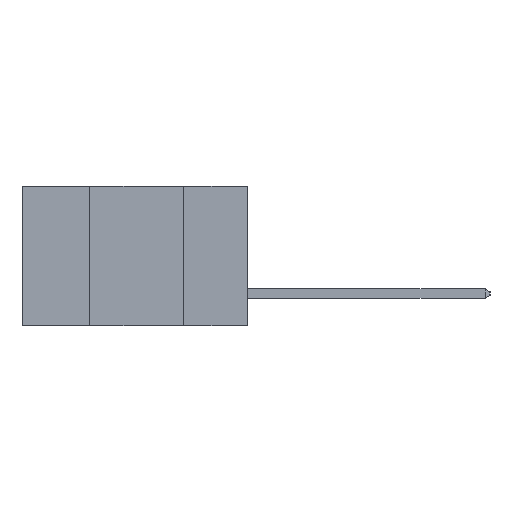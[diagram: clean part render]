
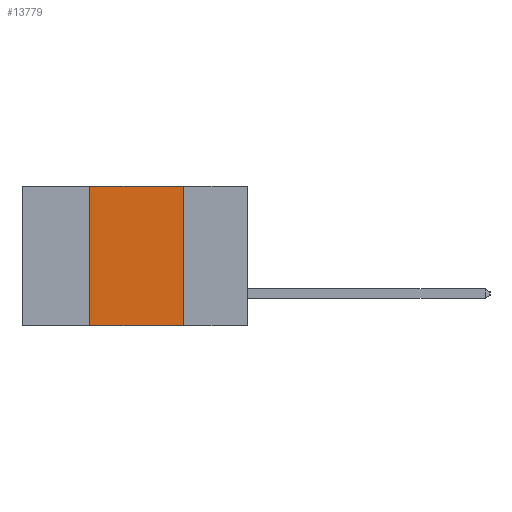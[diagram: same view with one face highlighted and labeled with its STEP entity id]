
A CAD part, left-side view. The second image highlights one B-rep face of the part: STEP entity #13779.
In plain terms, the highlighted planar face has unit normal (-1, 0, 0).
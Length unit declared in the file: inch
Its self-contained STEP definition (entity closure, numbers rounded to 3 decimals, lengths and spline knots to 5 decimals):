
#42 = CARTESIAN_POINT ( 'NONE',  ( 0., 0.42, 0. ) ) ;
#519 = CARTESIAN_POINT ( 'NONE',  ( 0., 0.17, -0.37 ) ) ;
#761 = EDGE_CURVE ( 'NONE', #22427, #6366, #16211, .T. ) ;
#766 = ORIENTED_EDGE ( 'NONE', *, *, #7990, .F. ) ;
#946 = LINE ( 'NONE', #19344, #10336 ) ;
#3542 = AXIS2_PLACEMENT_3D ( 'NONE', #10953, #18099, #7321 ) ;
#3591 = CARTESIAN_POINT ( 'NONE',  ( 0., 0.6, 0. ) ) ;
#4096 = VECTOR ( 'NONE', #5344, 39.37008 ) ;
#5140 = ORIENTED_EDGE ( 'NONE', *, *, #9234, .F. ) ;
#5344 = DIRECTION ( 'NONE',  ( 0., 0., -1. ) ) ;
#5467 = PLANE ( 'NONE',  #3542 ) ;
#5563 = DIRECTION ( 'NONE',  ( 0., 0., 1. ) ) ;
#5823 = ORIENTED_EDGE ( 'NONE', *, *, #761, .F. ) ;
#6366 = VERTEX_POINT ( 'NONE', #22508 ) ;
#6542 = DIRECTION ( 'NONE',  ( 0., -1., 0. ) ) ;
#6775 = EDGE_CURVE ( 'NONE', #22319, #14623, #946, .T. ) ;
#7321 = DIRECTION ( 'NONE',  ( 0., 0., -1. ) ) ;
#7990 = EDGE_CURVE ( 'NONE', #22319, #22427, #15069, .T. ) ;
#8758 = EDGE_LOOP ( 'NONE', ( #5140, #5823, #766, #14408 ) ) ;
#9030 = LINE ( 'NONE', #14471, #4096 ) ;
#9234 = EDGE_CURVE ( 'NONE', #6366, #14623, #9030, .T. ) ;
#10336 = VECTOR ( 'NONE', #19194, 39.37008 ) ;
#10953 = CARTESIAN_POINT ( 'NONE',  ( 0., 0.6, 0. ) ) ;
#11422 = VECTOR ( 'NONE', #6542, 39.37008 ) ;
#13779 = ADVANCED_FACE ( 'NONE', ( #19469 ), #5467, .F. ) ;
#14408 = ORIENTED_EDGE ( 'NONE', *, *, #6775, .T. ) ;
#14471 = CARTESIAN_POINT ( 'NONE',  ( 0., 0.17, 0. ) ) ;
#14623 = VERTEX_POINT ( 'NONE', #519 ) ;
#15069 = LINE ( 'NONE', #21683, #23190 ) ;
#16211 = LINE ( 'NONE', #3591, #11422 ) ;
#16331 = CARTESIAN_POINT ( 'NONE',  ( 0., 0.42, -0.37 ) ) ;
#18099 = DIRECTION ( 'NONE',  ( 1., 0., 0. ) ) ;
#19194 = DIRECTION ( 'NONE',  ( 0., -1., 0. ) ) ;
#19344 = CARTESIAN_POINT ( 'NONE',  ( 0., 0.6, -0.37 ) ) ;
#19469 = FACE_OUTER_BOUND ( 'NONE', #8758, .T. ) ;
#21683 = CARTESIAN_POINT ( 'NONE',  ( 0., 0.42, 0. ) ) ;
#22319 = VERTEX_POINT ( 'NONE', #16331 ) ;
#22427 = VERTEX_POINT ( 'NONE', #42 ) ;
#22508 = CARTESIAN_POINT ( 'NONE',  ( 0., 0.17, 0. ) ) ;
#23190 = VECTOR ( 'NONE', #5563, 39.37008 ) ;
